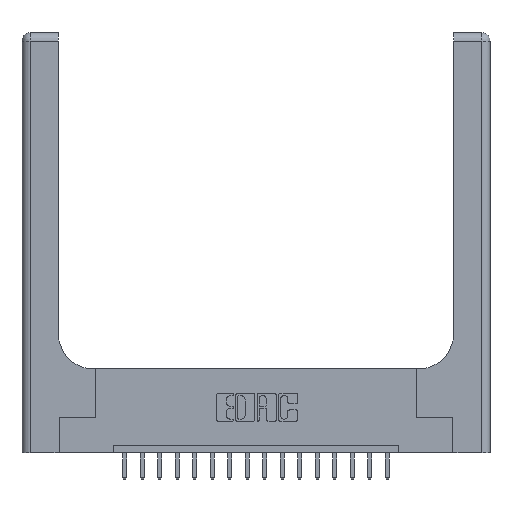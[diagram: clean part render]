
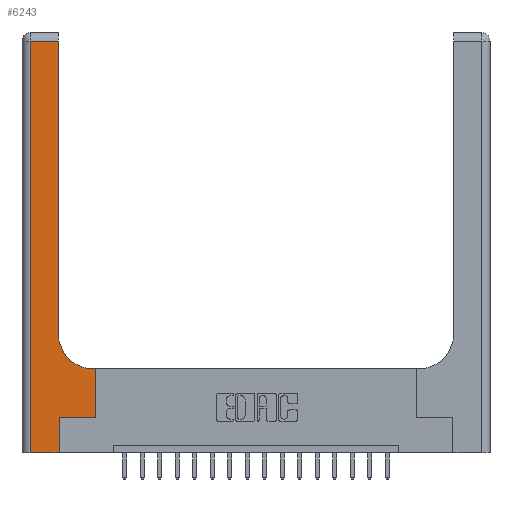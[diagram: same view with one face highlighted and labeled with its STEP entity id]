
A CAD part, top view. The second image highlights one B-rep face of the part: STEP entity #6243.
In plain terms, the highlighted planar face has unit normal (0, 0, 1).
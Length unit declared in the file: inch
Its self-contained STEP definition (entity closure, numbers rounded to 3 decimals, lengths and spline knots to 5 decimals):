
#170 = CARTESIAN_POINT ( 'NONE',  ( 0.265, 0.25, 0.37 ) ) ;
#1125 = LINE ( 'NONE', #16233, #3434 ) ;
#1308 = PLANE ( 'NONE',  #3202 ) ;
#1609 = CARTESIAN_POINT ( 'NONE',  ( 0.26, 0.85, 0.37 ) ) ;
#1662 = VECTOR ( 'NONE', #13926, 39.37008 ) ;
#2723 = ORIENTED_EDGE ( 'NONE', *, *, #6836, .T. ) ;
#2949 = DIRECTION ( 'NONE',  ( 0., 1., 0. ) ) ;
#2998 = VERTEX_POINT ( 'NONE', #10259 ) ;
#3202 = AXIS2_PLACEMENT_3D ( 'NONE', #13331, #18854, #7023 ) ;
#3216 = AXIS2_PLACEMENT_3D ( 'NONE', #13878, #18516, #13788 ) ;
#3368 = VERTEX_POINT ( 'NONE', #12778 ) ;
#3434 = VECTOR ( 'NONE', #2949, 39.37008 ) ;
#3714 = EDGE_CURVE ( 'NONE', #18994, #10215, #15544, .T. ) ;
#3786 = ORIENTED_EDGE ( 'NONE', *, *, #18686, .T. ) ;
#3913 = CARTESIAN_POINT ( 'NONE',  ( 0.265, 0., 0.37 ) ) ;
#3940 = ORIENTED_EDGE ( 'NONE', *, *, #17999, .T. ) ;
#4037 = CARTESIAN_POINT ( 'NONE',  ( 0.51, 0.6, 0.37 ) ) ;
#4208 = FACE_OUTER_BOUND ( 'NONE', #11382, .T. ) ;
#4258 = CARTESIAN_POINT ( 'NONE',  ( 0., 2.94, 0.37 ) ) ;
#4467 = VECTOR ( 'NONE', #19128, 39.37008 ) ;
#4572 = DIRECTION ( 'NONE',  ( 0., -1., 0. ) ) ;
#4590 = VERTEX_POINT ( 'NONE', #1609 ) ;
#4937 = EDGE_CURVE ( 'NONE', #10215, #2998, #14766, .T. ) ;
#5037 = EDGE_CURVE ( 'NONE', #2998, #15855, #15930, .T. ) ;
#5344 = ORIENTED_EDGE ( 'NONE', *, *, #3714, .T. ) ;
#5812 = VERTEX_POINT ( 'NONE', #16537 ) ;
#5954 = EDGE_CURVE ( 'NONE', #3368, #18994, #18269, .T. ) ;
#5998 = ORIENTED_EDGE ( 'NONE', *, *, #5954, .T. ) ;
#6029 = CARTESIAN_POINT ( 'NONE',  ( 0.06, 3., 0.37 ) ) ;
#6243 = ADVANCED_FACE ( 'NONE', ( #4208 ), #1308, .F. ) ;
#6286 = VECTOR ( 'NONE', #6725, 39.37008 ) ;
#6324 = CIRCLE ( 'NONE', #3216, 0.25 ) ;
#6725 = DIRECTION ( 'NONE',  ( 1., 0., 0. ) ) ;
#6836 = EDGE_CURVE ( 'NONE', #15855, #4590, #6324, .T. ) ;
#7023 = DIRECTION ( 'NONE',  ( -1., 0., 0. ) ) ;
#7169 = DIRECTION ( 'NONE',  ( -1., 0., 0. ) ) ;
#7478 = CARTESIAN_POINT ( 'NONE',  ( 0.528, 0.25, 0.37 ) ) ;
#8236 = ORIENTED_EDGE ( 'NONE', *, *, #4937, .T. ) ;
#9141 = DIRECTION ( 'NONE',  ( 1., 0., 0. ) ) ;
#9454 = VERTEX_POINT ( 'NONE', #16181 ) ;
#9481 = EDGE_CURVE ( 'NONE', #9454, #5812, #14369, .T. ) ;
#9659 = VECTOR ( 'NONE', #4572, 39.37008 ) ;
#10215 = VERTEX_POINT ( 'NONE', #7478 ) ;
#10259 = CARTESIAN_POINT ( 'NONE',  ( 0.528, 0.6, 0.37 ) ) ;
#10590 = LINE ( 'NONE', #16499, #16041 ) ;
#11382 = EDGE_LOOP ( 'NONE', ( #3940, #13781, #3786, #18264, #5998, #5344, #8236, #17839, #2723 ) ) ;
#11774 = CARTESIAN_POINT ( 'NONE',  ( 0.26, 0.6, 0.37 ) ) ;
#12289 = VECTOR ( 'NONE', #7169, 39.37008 ) ;
#12778 = CARTESIAN_POINT ( 'NONE',  ( 0.265, 0., 0.37 ) ) ;
#12849 = VECTOR ( 'NONE', #17672, 39.37008 ) ;
#13041 = CARTESIAN_POINT ( 'NONE',  ( 0.528, 0.25, 0.37 ) ) ;
#13331 = CARTESIAN_POINT ( 'NONE',  ( 0., 3., 0.37 ) ) ;
#13588 = EDGE_CURVE ( 'NONE', #15438, #3368, #10590, .T. ) ;
#13781 = ORIENTED_EDGE ( 'NONE', *, *, #9481, .T. ) ;
#13788 = DIRECTION ( 'NONE',  ( 1., 0., 0. ) ) ;
#13878 = CARTESIAN_POINT ( 'NONE',  ( 0.51, 0.85, 0.37 ) ) ;
#13926 = DIRECTION ( 'NONE',  ( 0., 1., 0. ) ) ;
#14107 = CARTESIAN_POINT ( 'NONE',  ( 0.265, 0.25, 0.37 ) ) ;
#14369 = LINE ( 'NONE', #4258, #12289 ) ;
#14766 = LINE ( 'NONE', #13041, #4467 ) ;
#14845 = LINE ( 'NONE', #6029, #9659 ) ;
#15438 = VERTEX_POINT ( 'NONE', #15885 ) ;
#15544 = LINE ( 'NONE', #14107, #6286 ) ;
#15855 = VERTEX_POINT ( 'NONE', #4037 ) ;
#15885 = CARTESIAN_POINT ( 'NONE',  ( 0.06, 0., 0.37 ) ) ;
#15930 = LINE ( 'NONE', #11774, #12849 ) ;
#16041 = VECTOR ( 'NONE', #9141, 39.37008 ) ;
#16181 = CARTESIAN_POINT ( 'NONE',  ( 0.26, 2.94, 0.37 ) ) ;
#16233 = CARTESIAN_POINT ( 'NONE',  ( 0.26, 3., 0.37 ) ) ;
#16499 = CARTESIAN_POINT ( 'NONE',  ( 0., 0., 0.37 ) ) ;
#16537 = CARTESIAN_POINT ( 'NONE',  ( 0.06, 2.94, 0.37 ) ) ;
#17672 = DIRECTION ( 'NONE',  ( -1., 0., 0. ) ) ;
#17839 = ORIENTED_EDGE ( 'NONE', *, *, #5037, .T. ) ;
#17999 = EDGE_CURVE ( 'NONE', #4590, #9454, #1125, .T. ) ;
#18264 = ORIENTED_EDGE ( 'NONE', *, *, #13588, .T. ) ;
#18269 = LINE ( 'NONE', #3913, #1662 ) ;
#18516 = DIRECTION ( 'NONE',  ( 0., 0., -1. ) ) ;
#18686 = EDGE_CURVE ( 'NONE', #5812, #15438, #14845, .T. ) ;
#18854 = DIRECTION ( 'NONE',  ( 0., 0., -1. ) ) ;
#18994 = VERTEX_POINT ( 'NONE', #170 ) ;
#19128 = DIRECTION ( 'NONE',  ( 0., 1., 0. ) ) ;
